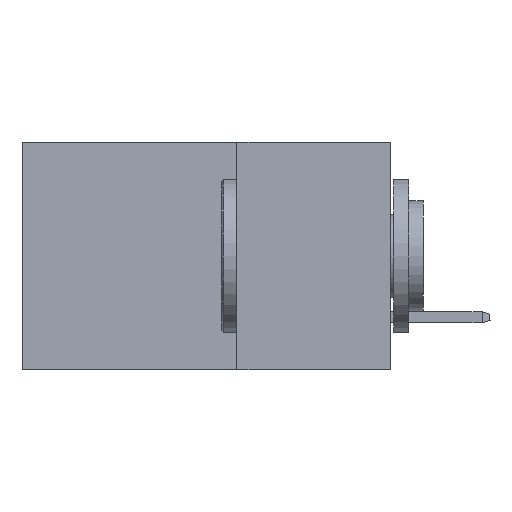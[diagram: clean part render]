
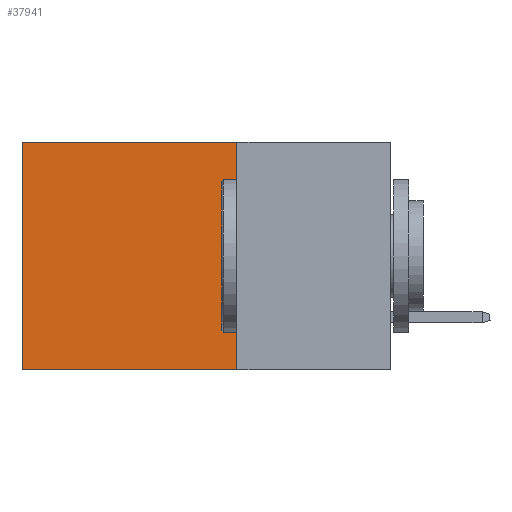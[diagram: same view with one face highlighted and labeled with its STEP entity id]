
A CAD part, left-side view. The second image highlights one B-rep face of the part: STEP entity #37941.
In plain terms, the highlighted planar face has unit normal (-1, 0, 0).
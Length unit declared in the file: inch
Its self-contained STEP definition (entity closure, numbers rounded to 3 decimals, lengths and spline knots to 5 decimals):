
#1930 = CARTESIAN_POINT ( 'NONE',  ( 0.2875, 0.6, 0. ) ) ;
#3421 = VECTOR ( 'NONE', #8491, 39.37008 ) ;
#3867 = DIRECTION ( 'NONE',  ( 0., 0., -1. ) ) ;
#5112 = LINE ( 'NONE', #21627, #28617 ) ;
#6005 = DIRECTION ( 'NONE',  ( 0., 1., 0. ) ) ;
#6605 = DIRECTION ( 'NONE',  ( 0., 1., 0. ) ) ;
#7052 = CARTESIAN_POINT ( 'NONE',  ( 0.2875, 0.25, 0. ) ) ;
#7414 = VERTEX_POINT ( 'NONE', #1930 ) ;
#8491 = DIRECTION ( 'NONE',  ( 0., 0., -1. ) ) ;
#9246 = VECTOR ( 'NONE', #3867, 39.37008 ) ;
#9486 = FACE_OUTER_BOUND ( 'NONE', #35850, .T. ) ;
#13671 = EDGE_CURVE ( 'NONE', #7414, #28274, #38955, .T. ) ;
#14145 = VERTEX_POINT ( 'NONE', #25452 ) ;
#16202 = ORIENTED_EDGE ( 'NONE', *, *, #13671, .T. ) ;
#19037 = DIRECTION ( 'NONE',  ( 0., 0., -1. ) ) ;
#19559 = DIRECTION ( 'NONE',  ( 1., 0., 0. ) ) ;
#20957 = AXIS2_PLACEMENT_3D ( 'NONE', #22257, #19559, #19037 ) ;
#21537 = ORIENTED_EDGE ( 'NONE', *, *, #32667, .F. ) ;
#21627 = CARTESIAN_POINT ( 'NONE',  ( 0.2875, 0.25, 0. ) ) ;
#22257 = CARTESIAN_POINT ( 'NONE',  ( 0.2875, 0.25, 0. ) ) ;
#22340 = VECTOR ( 'NONE', #6605, 39.37008 ) ;
#22580 = EDGE_CURVE ( 'NONE', #14145, #28274, #32445, .T. ) ;
#23254 = CARTESIAN_POINT ( 'NONE',  ( 0.2875, 0.6, 0. ) ) ;
#23590 = ORIENTED_EDGE ( 'NONE', *, *, #22580, .F. ) ;
#23696 = ORIENTED_EDGE ( 'NONE', *, *, #30960, .T. ) ;
#25452 = CARTESIAN_POINT ( 'NONE',  ( 0.2875, 0.25, -0.37 ) ) ;
#28274 = VERTEX_POINT ( 'NONE', #28876 ) ;
#28617 = VECTOR ( 'NONE', #6005, 39.37008 ) ;
#28876 = CARTESIAN_POINT ( 'NONE',  ( 0.2875, 0.6, -0.37 ) ) ;
#30897 = VERTEX_POINT ( 'NONE', #36047 ) ;
#30960 = EDGE_CURVE ( 'NONE', #30897, #7414, #5112, .T. ) ;
#31408 = PLANE ( 'NONE',  #20957 ) ;
#32445 = LINE ( 'NONE', #36795, #22340 ) ;
#32667 = EDGE_CURVE ( 'NONE', #30897, #14145, #39501, .T. ) ;
#35850 = EDGE_LOOP ( 'NONE', ( #16202, #23590, #21537, #23696 ) ) ;
#36047 = CARTESIAN_POINT ( 'NONE',  ( 0.2875, 0.25, 0. ) ) ;
#36795 = CARTESIAN_POINT ( 'NONE',  ( 0.2875, 0.25, -0.37 ) ) ;
#37941 = ADVANCED_FACE ( 'NONE', ( #9486 ), #31408, .F. ) ;
#38955 = LINE ( 'NONE', #23254, #3421 ) ;
#39501 = LINE ( 'NONE', #7052, #9246 ) ;
